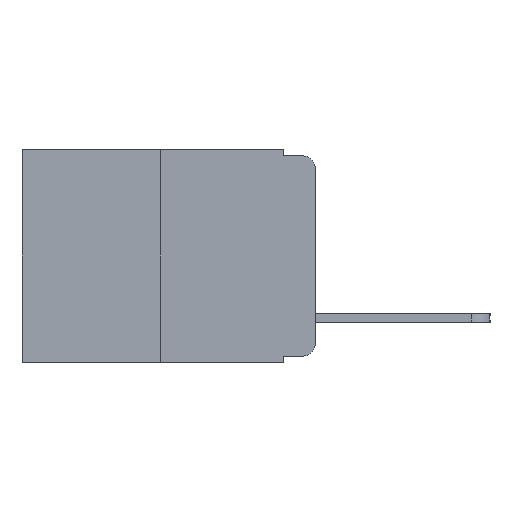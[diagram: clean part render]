
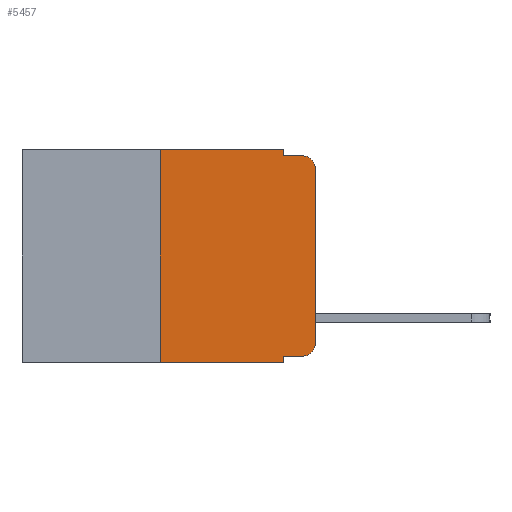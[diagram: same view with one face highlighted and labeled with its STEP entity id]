
A CAD part, left-side view. The second image highlights one B-rep face of the part: STEP entity #5457.
In plain terms, the highlighted planar face has unit normal (-1, 0, 0).
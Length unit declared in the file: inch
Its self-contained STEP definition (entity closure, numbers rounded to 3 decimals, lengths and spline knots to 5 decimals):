
#79 = EDGE_CURVE ( 'NONE', #4928, #1386, #8854, .T. ) ;
#356 = DIRECTION ( 'NONE',  ( -1., 0., 0. ) ) ;
#674 = LINE ( 'NONE', #8836, #6869 ) ;
#796 = CARTESIAN_POINT ( 'NONE',  ( 0., 0.02, -0.333 ) ) ;
#902 = VERTEX_POINT ( 'NONE', #3943 ) ;
#1008 = LINE ( 'NONE', #3368, #6478 ) ;
#1152 = EDGE_CURVE ( 'NONE', #14765, #5843, #10932, .T. ) ;
#1180 = DIRECTION ( 'NONE',  ( 0., 0., 1. ) ) ;
#1338 = CARTESIAN_POINT ( 'NONE',  ( 0., 0., -0.313 ) ) ;
#1386 = VERTEX_POINT ( 'NONE', #11737 ) ;
#1641 = CARTESIAN_POINT ( 'NONE',  ( 0., 0., -0.03 ) ) ;
#1681 = DIRECTION ( 'NONE',  ( 0., 0., -1. ) ) ;
#1776 = EDGE_LOOP ( 'NONE', ( #10988, #5212, #9757, #10817, #9243, #4495, #9423, #10835, #12289, #1788 ) ) ;
#1788 = ORIENTED_EDGE ( 'NONE', *, *, #5126, .T. ) ;
#1848 = DIRECTION ( 'NONE',  ( 0., -1., 0. ) ) ;
#2760 = DIRECTION ( 'NONE',  ( 0., -1., 0. ) ) ;
#2838 = LINE ( 'NONE', #10375, #5938 ) ;
#2900 = DIRECTION ( 'NONE',  ( 0., 0., -1. ) ) ;
#3326 = FACE_OUTER_BOUND ( 'NONE', #1776, .T. ) ;
#3368 = CARTESIAN_POINT ( 'NONE',  ( 0., 0.051, 0. ) ) ;
#3714 = CARTESIAN_POINT ( 'NONE',  ( 0., 0.473, -0.343 ) ) ;
#3943 = CARTESIAN_POINT ( 'NONE',  ( 0., 0.051, -0.333 ) ) ;
#4338 = DIRECTION ( 'NONE',  ( -1., 0., 0. ) ) ;
#4495 = ORIENTED_EDGE ( 'NONE', *, *, #10018, .F. ) ;
#4561 = DIRECTION ( 'NONE',  ( 0., -1., 0. ) ) ;
#4928 = VERTEX_POINT ( 'NONE', #1641 ) ;
#5100 = CARTESIAN_POINT ( 'NONE',  ( 0., 0.473, 0. ) ) ;
#5126 = EDGE_CURVE ( 'NONE', #7399, #11864, #10764, .T. ) ;
#5212 = ORIENTED_EDGE ( 'NONE', *, *, #79, .T. ) ;
#5457 = ADVANCED_FACE ( 'NONE', ( #3326 ), #12051, .F. ) ;
#5625 = DIRECTION ( 'NONE',  ( 0., 0., -1. ) ) ;
#5638 = DIRECTION ( 'NONE',  ( 0., 0., 1. ) ) ;
#5687 = CARTESIAN_POINT ( 'NONE',  ( 0., 0.051, -0.333 ) ) ;
#5799 = AXIS2_PLACEMENT_3D ( 'NONE', #11268, #4338, #12423 ) ;
#5843 = VERTEX_POINT ( 'NONE', #12696 ) ;
#5938 = VECTOR ( 'NONE', #1180, 39.37008 ) ;
#6226 = VERTEX_POINT ( 'NONE', #6570 ) ;
#6229 = VECTOR ( 'NONE', #5638, 39.37008 ) ;
#6332 = CARTESIAN_POINT ( 'NONE',  ( 0., 0.473, 0. ) ) ;
#6478 = VECTOR ( 'NONE', #8073, 39.37008 ) ;
#6570 = CARTESIAN_POINT ( 'NONE',  ( 0., 0.25, -0.343 ) ) ;
#6822 = EDGE_CURVE ( 'NONE', #11864, #4928, #9329, .T. ) ;
#6869 = VECTOR ( 'NONE', #1848, 39.37008 ) ;
#7090 = CARTESIAN_POINT ( 'NONE',  ( 0., 0.02, -0.03 ) ) ;
#7399 = VERTEX_POINT ( 'NONE', #796 ) ;
#7413 = VERTEX_POINT ( 'NONE', #11236 ) ;
#7770 = EDGE_CURVE ( 'NONE', #6226, #10228, #9830, .T. ) ;
#7912 = VECTOR ( 'NONE', #5625, 39.37008 ) ;
#8030 = VECTOR ( 'NONE', #4561, 39.37008 ) ;
#8073 = DIRECTION ( 'NONE',  ( 0., 0., -1. ) ) ;
#8284 = VECTOR ( 'NONE', #2760, 39.37008 ) ;
#8655 = LINE ( 'NONE', #5100, #8284 ) ;
#8691 = DIRECTION ( 'NONE',  ( 1., 0., 0. ) ) ;
#8705 = CARTESIAN_POINT ( 'NONE',  ( 0., 0.051, 0. ) ) ;
#8836 = CARTESIAN_POINT ( 'NONE',  ( 0., 0.051, -0.01 ) ) ;
#8854 = CIRCLE ( 'NONE', #9589, 0.02 ) ;
#9243 = ORIENTED_EDGE ( 'NONE', *, *, #14739, .F. ) ;
#9329 = LINE ( 'NONE', #10259, #6229 ) ;
#9423 = ORIENTED_EDGE ( 'NONE', *, *, #7770, .T. ) ;
#9589 = AXIS2_PLACEMENT_3D ( 'NONE', #7090, #356, #2900 ) ;
#9622 = DIRECTION ( 'NONE',  ( 0., -1., 0. ) ) ;
#9718 = EDGE_CURVE ( 'NONE', #5843, #1386, #674, .T. ) ;
#9757 = ORIENTED_EDGE ( 'NONE', *, *, #9718, .F. ) ;
#9830 = LINE ( 'NONE', #3714, #12506 ) ;
#10018 = EDGE_CURVE ( 'NONE', #6226, #7413, #2838, .T. ) ;
#10228 = VERTEX_POINT ( 'NONE', #10790 ) ;
#10259 = CARTESIAN_POINT ( 'NONE',  ( 0., 0., 0. ) ) ;
#10375 = CARTESIAN_POINT ( 'NONE',  ( 0., 0.25, 0. ) ) ;
#10570 = EDGE_CURVE ( 'NONE', #902, #7399, #11059, .T. ) ;
#10764 = CIRCLE ( 'NONE', #5799, 0.02 ) ;
#10790 = CARTESIAN_POINT ( 'NONE',  ( 0., 0.051, -0.343 ) ) ;
#10817 = ORIENTED_EDGE ( 'NONE', *, *, #1152, .F. ) ;
#10835 = ORIENTED_EDGE ( 'NONE', *, *, #13337, .F. ) ;
#10932 = LINE ( 'NONE', #12239, #7912 ) ;
#10988 = ORIENTED_EDGE ( 'NONE', *, *, #6822, .T. ) ;
#11059 = LINE ( 'NONE', #5687, #8030 ) ;
#11236 = CARTESIAN_POINT ( 'NONE',  ( 0., 0.25, 0. ) ) ;
#11268 = CARTESIAN_POINT ( 'NONE',  ( 0., 0.02, -0.313 ) ) ;
#11737 = CARTESIAN_POINT ( 'NONE',  ( 0., 0.02, -0.01 ) ) ;
#11864 = VERTEX_POINT ( 'NONE', #1338 ) ;
#12051 = PLANE ( 'NONE',  #14729 ) ;
#12239 = CARTESIAN_POINT ( 'NONE',  ( 0., 0.051, 0. ) ) ;
#12289 = ORIENTED_EDGE ( 'NONE', *, *, #10570, .T. ) ;
#12423 = DIRECTION ( 'NONE',  ( 0., 0., -1. ) ) ;
#12506 = VECTOR ( 'NONE', #9622, 39.37008 ) ;
#12696 = CARTESIAN_POINT ( 'NONE',  ( 0., 0.051, -0.01 ) ) ;
#13337 = EDGE_CURVE ( 'NONE', #902, #10228, #1008, .T. ) ;
#14729 = AXIS2_PLACEMENT_3D ( 'NONE', #6332, #8691, #1681 ) ;
#14739 = EDGE_CURVE ( 'NONE', #7413, #14765, #8655, .T. ) ;
#14765 = VERTEX_POINT ( 'NONE', #8705 ) ;
